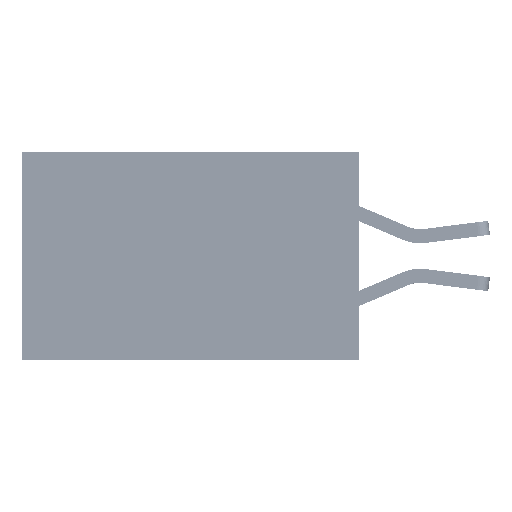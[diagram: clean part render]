
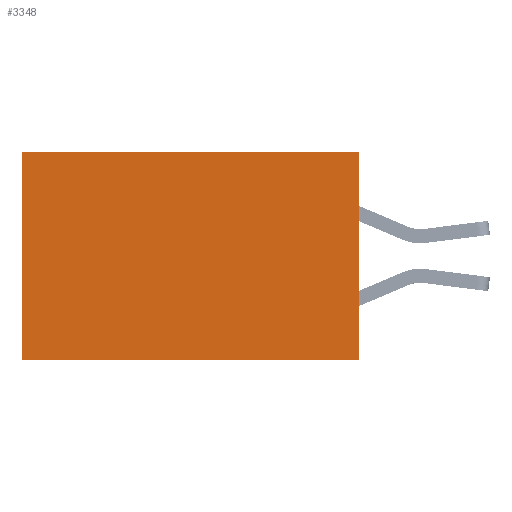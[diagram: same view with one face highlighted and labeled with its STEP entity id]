
A CAD part, left-side view. The second image highlights one B-rep face of the part: STEP entity #3348.
In plain terms, the highlighted planar face has unit normal (-1, 0, 0).
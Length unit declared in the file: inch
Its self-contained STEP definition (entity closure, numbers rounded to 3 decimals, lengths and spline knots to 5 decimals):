
#679 = CARTESIAN_POINT ( 'NONE',  ( 0.2875, 0.6, -0.37 ) ) ;
#3031 = CARTESIAN_POINT ( 'NONE',  ( 0.2875, 0., 0. ) ) ;
#3348 = ADVANCED_FACE ( 'NONE', ( #37307 ), #44140, .F. ) ;
#3466 = CARTESIAN_POINT ( 'NONE',  ( 0.2875, 0., -0.37 ) ) ;
#3475 = CARTESIAN_POINT ( 'NONE',  ( 0.2875, 0.6, 0. ) ) ;
#3535 = CARTESIAN_POINT ( 'NONE',  ( 0.2875, 0.6, 0. ) ) ;
#10222 = LINE ( 'NONE', #43834, #25925 ) ;
#10959 = LINE ( 'NONE', #46381, #42268 ) ;
#11151 = DIRECTION ( 'NONE',  ( 0., 0., -1. ) ) ;
#11167 = DIRECTION ( 'NONE',  ( 0., 0., -1. ) ) ;
#17424 = DIRECTION ( 'NONE',  ( 0., 1., 0. ) ) ;
#21953 = VECTOR ( 'NONE', #17424, 39.37008 ) ;
#23627 = VECTOR ( 'NONE', #11167, 39.37008 ) ;
#25925 = VECTOR ( 'NONE', #11151, 39.37008 ) ;
#26507 = EDGE_CURVE ( 'NONE', #37688, #47514, #40440, .T. ) ;
#27959 = VERTEX_POINT ( 'NONE', #29893 ) ;
#29292 = DIRECTION ( 'NONE',  ( 0., 0., -1. ) ) ;
#29893 = CARTESIAN_POINT ( 'NONE',  ( 0.2875, 0., 0. ) ) ;
#30245 = ORIENTED_EDGE ( 'NONE', *, *, #39808, .T. ) ;
#31203 = EDGE_CURVE ( 'NONE', #27959, #37970, #10959, .T. ) ;
#32693 = DIRECTION ( 'NONE',  ( 1., 0., 0. ) ) ;
#32832 = EDGE_CURVE ( 'NONE', #27959, #37688, #10222, .T. ) ;
#34209 = EDGE_LOOP ( 'NONE', ( #30245, #39124, #35656, #44880 ) ) ;
#34626 = CARTESIAN_POINT ( 'NONE',  ( 0.2875, 0., -0.37 ) ) ;
#35656 = ORIENTED_EDGE ( 'NONE', *, *, #32832, .F. ) ;
#35713 = DIRECTION ( 'NONE',  ( 0., 1., 0. ) ) ;
#37307 = FACE_OUTER_BOUND ( 'NONE', #34209, .T. ) ;
#37688 = VERTEX_POINT ( 'NONE', #34626 ) ;
#37970 = VERTEX_POINT ( 'NONE', #3475 ) ;
#39124 = ORIENTED_EDGE ( 'NONE', *, *, #26507, .F. ) ;
#39808 = EDGE_CURVE ( 'NONE', #37970, #47514, #47897, .T. ) ;
#40440 = LINE ( 'NONE', #3466, #21953 ) ;
#42027 = AXIS2_PLACEMENT_3D ( 'NONE', #3031, #32693, #29292 ) ;
#42268 = VECTOR ( 'NONE', #35713, 39.37008 ) ;
#43834 = CARTESIAN_POINT ( 'NONE',  ( 0.2875, 0., 0. ) ) ;
#44140 = PLANE ( 'NONE',  #42027 ) ;
#44880 = ORIENTED_EDGE ( 'NONE', *, *, #31203, .T. ) ;
#46381 = CARTESIAN_POINT ( 'NONE',  ( 0.2875, 0., 0. ) ) ;
#47514 = VERTEX_POINT ( 'NONE', #679 ) ;
#47897 = LINE ( 'NONE', #3535, #23627 ) ;
